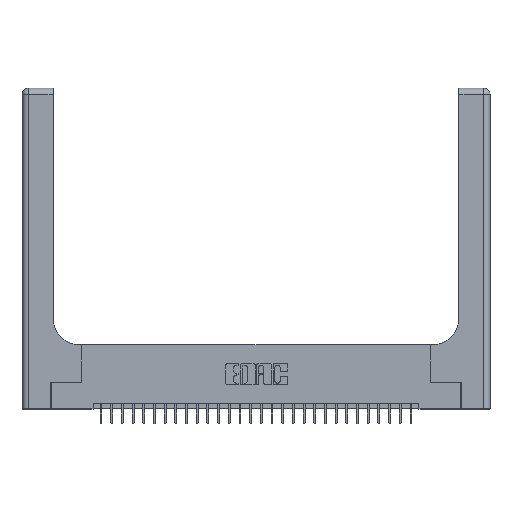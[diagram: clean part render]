
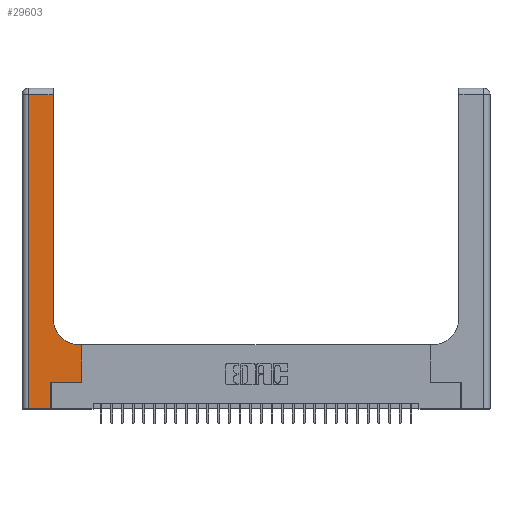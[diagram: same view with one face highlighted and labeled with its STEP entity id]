
A CAD part, top view. The second image highlights one B-rep face of the part: STEP entity #29603.
In plain terms, the highlighted planar face has unit normal (0, 0, 1).
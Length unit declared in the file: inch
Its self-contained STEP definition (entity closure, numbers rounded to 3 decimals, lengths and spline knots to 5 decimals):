
#861 = LINE ( 'NONE', #18882, #29828 ) ;
#1371 = ORIENTED_EDGE ( 'NONE', *, *, #10032, .T. ) ;
#1372 = EDGE_CURVE ( 'NONE', #25864, #13503, #29945, .T. ) ;
#1697 = EDGE_CURVE ( 'NONE', #13503, #3382, #8640, .T. ) ;
#1989 = VECTOR ( 'NONE', #28528, 39.37008 ) ;
#2018 = DIRECTION ( 'NONE',  ( -1., 0., 0. ) ) ;
#2300 = DIRECTION ( 'NONE',  ( -1., 0., 0. ) ) ;
#2366 = DIRECTION ( 'NONE',  ( 1., 0., 0. ) ) ;
#2404 = LINE ( 'NONE', #29548, #14197 ) ;
#2522 = DIRECTION ( 'NONE',  ( 0., 0., -1. ) ) ;
#3382 = VERTEX_POINT ( 'NONE', #26044 ) ;
#3834 = DIRECTION ( 'NONE',  ( 0., 1., 0. ) ) ;
#4129 = ORIENTED_EDGE ( 'NONE', *, *, #25339, .T. ) ;
#4441 = VECTOR ( 'NONE', #29483, 39.37008 ) ;
#4890 = ORIENTED_EDGE ( 'NONE', *, *, #27440, .T. ) ;
#5229 = DIRECTION ( 'NONE',  ( 0., 0., -1. ) ) ;
#5433 = CARTESIAN_POINT ( 'NONE',  ( 0.06, 2.94, 0.37 ) ) ;
#6895 = ORIENTED_EDGE ( 'NONE', *, *, #1697, .T. ) ;
#7528 = FACE_OUTER_BOUND ( 'NONE', #21030, .T. ) ;
#8024 = CARTESIAN_POINT ( 'NONE',  ( 0.06, 0., 0.37 ) ) ;
#8640 = LINE ( 'NONE', #15576, #19688 ) ;
#8652 = CARTESIAN_POINT ( 'NONE',  ( 0.269, 0.25, 0.37 ) ) ;
#9908 = DIRECTION ( 'NONE',  ( 0., 1., 0. ) ) ;
#10032 = EDGE_CURVE ( 'NONE', #3382, #23803, #18909, .T. ) ;
#10510 = DIRECTION ( 'NONE',  ( 0., 1., 0. ) ) ;
#10740 = VECTOR ( 'NONE', #2018, 39.37008 ) ;
#12053 = LINE ( 'NONE', #26384, #14166 ) ;
#12107 = DIRECTION ( 'NONE',  ( 0., -1., 0. ) ) ;
#13425 = EDGE_CURVE ( 'NONE', #23803, #14767, #13558, .T. ) ;
#13503 = VERTEX_POINT ( 'NONE', #28089 ) ;
#13558 = CIRCLE ( 'NONE', #26862, 0.25 ) ;
#14166 = VECTOR ( 'NONE', #9908, 39.37008 ) ;
#14197 = VECTOR ( 'NONE', #3834, 39.37008 ) ;
#14613 = DIRECTION ( 'NONE',  ( -1., 0., 0. ) ) ;
#14767 = VERTEX_POINT ( 'NONE', #24659 ) ;
#15576 = CARTESIAN_POINT ( 'NONE',  ( 0.5585, 0.25, 0.37 ) ) ;
#16544 = CARTESIAN_POINT ( 'NONE',  ( 0.269, 0., 0.37 ) ) ;
#16564 = EDGE_CURVE ( 'NONE', #14767, #21590, #12053, .T. ) ;
#16652 = AXIS2_PLACEMENT_3D ( 'NONE', #24147, #5229, #14613 ) ;
#16814 = CARTESIAN_POINT ( 'NONE',  ( 0., 0., 0.37 ) ) ;
#16948 = VECTOR ( 'NONE', #2300, 39.37008 ) ;
#18677 = VERTEX_POINT ( 'NONE', #8024 ) ;
#18882 = CARTESIAN_POINT ( 'NONE',  ( 0.06, 3., 0.37 ) ) ;
#18909 = LINE ( 'NONE', #23374, #16948 ) ;
#19636 = CARTESIAN_POINT ( 'NONE',  ( 0.2915, 2.94, 0.37 ) ) ;
#19688 = VECTOR ( 'NONE', #10510, 39.37008 ) ;
#21030 = EDGE_LOOP ( 'NONE', ( #26165, #4890, #4129, #28699, #27779, #27791, #6895, #1371, #24938 ) ) ;
#21083 = EDGE_CURVE ( 'NONE', #18677, #21889, #25738, .T. ) ;
#21590 = VERTEX_POINT ( 'NONE', #19636 ) ;
#21889 = VERTEX_POINT ( 'NONE', #16544 ) ;
#23085 = LINE ( 'NONE', #25402, #10740 ) ;
#23374 = CARTESIAN_POINT ( 'NONE',  ( 0.2915, 0.6, 0.37 ) ) ;
#23743 = CARTESIAN_POINT ( 'NONE',  ( 0.5415, 0.85, 0.37 ) ) ;
#23803 = VERTEX_POINT ( 'NONE', #26370 ) ;
#24147 = CARTESIAN_POINT ( 'NONE',  ( 0., 3., 0.37 ) ) ;
#24659 = CARTESIAN_POINT ( 'NONE',  ( 0.2915, 0.85, 0.37 ) ) ;
#24938 = ORIENTED_EDGE ( 'NONE', *, *, #13425, .T. ) ;
#25339 = EDGE_CURVE ( 'NONE', #27179, #18677, #861, .T. ) ;
#25402 = CARTESIAN_POINT ( 'NONE',  ( 0., 2.94, 0.37 ) ) ;
#25738 = LINE ( 'NONE', #16814, #1989 ) ;
#25864 = VERTEX_POINT ( 'NONE', #8652 ) ;
#26044 = CARTESIAN_POINT ( 'NONE',  ( 0.5585, 0.6, 0.37 ) ) ;
#26165 = ORIENTED_EDGE ( 'NONE', *, *, #16564, .T. ) ;
#26315 = PLANE ( 'NONE',  #16652 ) ;
#26370 = CARTESIAN_POINT ( 'NONE',  ( 0.5415, 0.6, 0.37 ) ) ;
#26384 = CARTESIAN_POINT ( 'NONE',  ( 0.2915, 3., 0.37 ) ) ;
#26862 = AXIS2_PLACEMENT_3D ( 'NONE', #23743, #2522, #2366 ) ;
#26880 = CARTESIAN_POINT ( 'NONE',  ( 0.269, 0.25, 0.37 ) ) ;
#27179 = VERTEX_POINT ( 'NONE', #5433 ) ;
#27440 = EDGE_CURVE ( 'NONE', #21590, #27179, #23085, .T. ) ;
#27745 = EDGE_CURVE ( 'NONE', #21889, #25864, #2404, .T. ) ;
#27779 = ORIENTED_EDGE ( 'NONE', *, *, #27745, .T. ) ;
#27791 = ORIENTED_EDGE ( 'NONE', *, *, #1372, .T. ) ;
#28089 = CARTESIAN_POINT ( 'NONE',  ( 0.5585, 0.25, 0.37 ) ) ;
#28528 = DIRECTION ( 'NONE',  ( 1., 0., 0. ) ) ;
#28699 = ORIENTED_EDGE ( 'NONE', *, *, #21083, .T. ) ;
#29483 = DIRECTION ( 'NONE',  ( 1., 0., 0. ) ) ;
#29548 = CARTESIAN_POINT ( 'NONE',  ( 0.269, 0., 0.37 ) ) ;
#29603 = ADVANCED_FACE ( 'NONE', ( #7528 ), #26315, .F. ) ;
#29828 = VECTOR ( 'NONE', #12107, 39.37008 ) ;
#29945 = LINE ( 'NONE', #26880, #4441 ) ;
